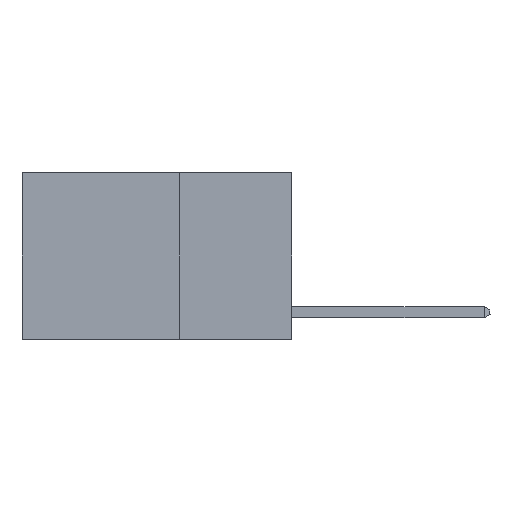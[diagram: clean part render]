
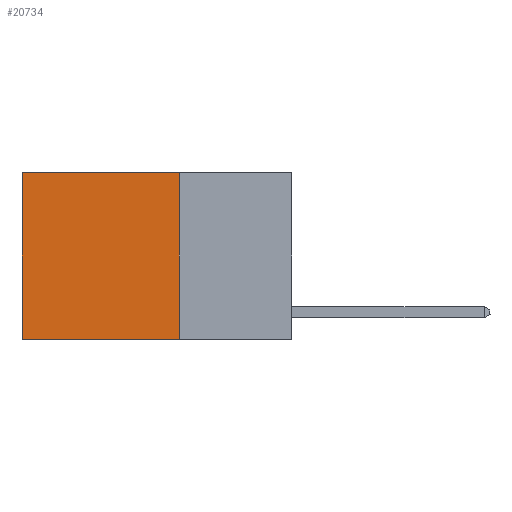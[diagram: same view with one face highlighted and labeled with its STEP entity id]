
A CAD part, left-side view. The second image highlights one B-rep face of the part: STEP entity #20734.
In plain terms, the highlighted planar face has unit normal (-1, 0, 0).
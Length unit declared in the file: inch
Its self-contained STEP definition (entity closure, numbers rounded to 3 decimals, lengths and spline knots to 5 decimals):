
#924 = VECTOR ( 'NONE', #22133, 39.37008 ) ;
#1203 = FACE_OUTER_BOUND ( 'NONE', #29865, .T. ) ;
#1416 = CARTESIAN_POINT ( 'NONE',  ( 0.2625, 0.6, -0.37 ) ) ;
#1517 = VECTOR ( 'NONE', #19405, 39.37008 ) ;
#1901 = VERTEX_POINT ( 'NONE', #16720 ) ;
#1984 = LINE ( 'NONE', #19791, #924 ) ;
#3602 = CARTESIAN_POINT ( 'NONE',  ( 0.2625, 0.25, 0. ) ) ;
#4289 = VERTEX_POINT ( 'NONE', #1416 ) ;
#6034 = CARTESIAN_POINT ( 'NONE',  ( 0.2625, 0.6, 0. ) ) ;
#9273 = CARTESIAN_POINT ( 'NONE',  ( 0.2625, 0.25, 0. ) ) ;
#9463 = AXIS2_PLACEMENT_3D ( 'NONE', #16783, #23546, #16877 ) ;
#9885 = ORIENTED_EDGE ( 'NONE', *, *, #12487, .T. ) ;
#12024 = VERTEX_POINT ( 'NONE', #16152 ) ;
#12487 = EDGE_CURVE ( 'NONE', #19130, #4289, #29695, .T. ) ;
#16152 = CARTESIAN_POINT ( 'NONE',  ( 0.2625, 0.25, -0.37 ) ) ;
#16720 = CARTESIAN_POINT ( 'NONE',  ( 0.2625, 0.25, 0. ) ) ;
#16783 = CARTESIAN_POINT ( 'NONE',  ( 0.2625, 0.25, 0. ) ) ;
#16877 = DIRECTION ( 'NONE',  ( 0., 0., -1. ) ) ;
#17052 = CARTESIAN_POINT ( 'NONE',  ( 0.2625, 0.6, 0. ) ) ;
#18780 = DIRECTION ( 'NONE',  ( 0., 0., -1. ) ) ;
#19130 = VERTEX_POINT ( 'NONE', #6034 ) ;
#19405 = DIRECTION ( 'NONE',  ( 0., 0., -1. ) ) ;
#19473 = EDGE_CURVE ( 'NONE', #12024, #4289, #1984, .T. ) ;
#19791 = CARTESIAN_POINT ( 'NONE',  ( 0.2625, 0.25, -0.37 ) ) ;
#19928 = EDGE_CURVE ( 'NONE', #1901, #12024, #26206, .T. ) ;
#20622 = PLANE ( 'NONE',  #9463 ) ;
#20734 = ADVANCED_FACE ( 'NONE', ( #1203 ), #20622, .F. ) ;
#20917 = VECTOR ( 'NONE', #24394, 39.37008 ) ;
#22133 = DIRECTION ( 'NONE',  ( 0., 1., 0. ) ) ;
#22494 = ORIENTED_EDGE ( 'NONE', *, *, #27219, .T. ) ;
#23433 = LINE ( 'NONE', #3602, #20917 ) ;
#23546 = DIRECTION ( 'NONE',  ( 1., 0., 0. ) ) ;
#24394 = DIRECTION ( 'NONE',  ( 0., 1., 0. ) ) ;
#24396 = VECTOR ( 'NONE', #18780, 39.37008 ) ;
#25881 = ORIENTED_EDGE ( 'NONE', *, *, #19928, .F. ) ;
#25903 = ORIENTED_EDGE ( 'NONE', *, *, #19473, .F. ) ;
#26206 = LINE ( 'NONE', #9273, #24396 ) ;
#27219 = EDGE_CURVE ( 'NONE', #1901, #19130, #23433, .T. ) ;
#29695 = LINE ( 'NONE', #17052, #1517 ) ;
#29865 = EDGE_LOOP ( 'NONE', ( #9885, #25903, #25881, #22494 ) ) ;
